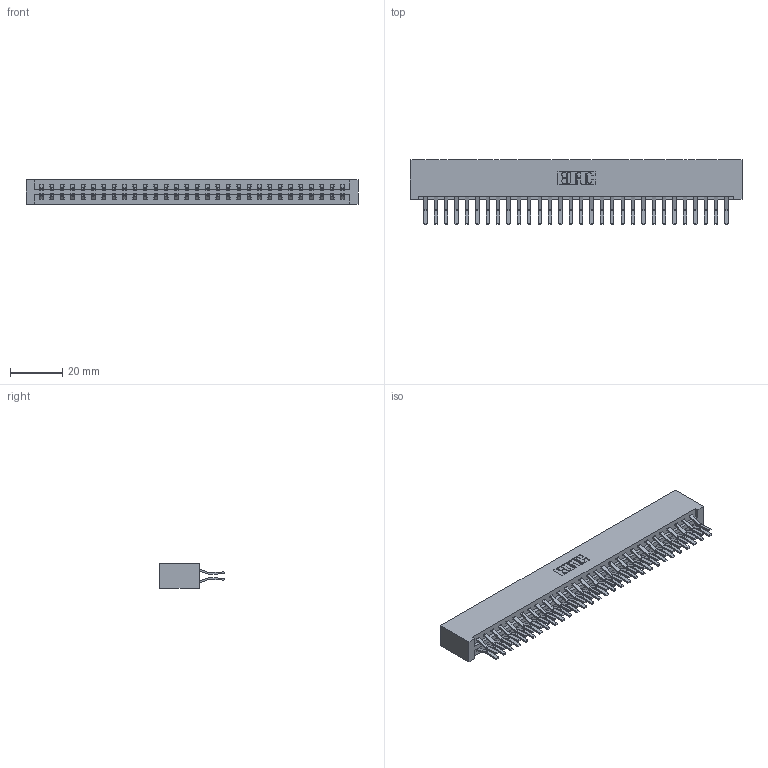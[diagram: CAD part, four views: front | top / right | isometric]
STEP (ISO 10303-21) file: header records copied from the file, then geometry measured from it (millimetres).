
FILE_DESCRIPTION (( 'STEP AP203' ), '1' );
FILE_NAME ('337-060-560-201.STEP', '2019-10-09T20:54:15', ( '' ), ( '' ), 'SwSTEP 2.0', 'SolidWorks 2016', '' );
FILE_SCHEMA (( 'CONFIG_CONTROL_DESIGN' ));
Length unit declared in the file: inch
Products named in the file (3): 337-060-560-201; 345-292-001_560 Tail; 337 Part_No Mounting Lugs
Assembly tree (61 placements, depth 2):
  337-060-560-201
    337 Part_No Mounting Lugs
    345-292-001_560 Tail  x60
Bounding box: 126.75 x 24.78 x 9.4 mm (x, y, z)
Volume: 14351.8 mm3; surface area: 17302.5 mm2
Topology: 61 solids, 61 shells, 3466 faces, 10307 edges, 6790 vertices
Faces by surface type: plane 2346, cylinder 1120
Entity records: 24623 total; most frequent: CARTESIAN_POINT 4158, ORIENTED_EDGE 4094, DIRECTION 3555, EDGE_CURVE 2047, LINE 1923, VECTOR 1923, VERTEX_POINT 1362, AXIS2_PLACEMENT_3D 816
